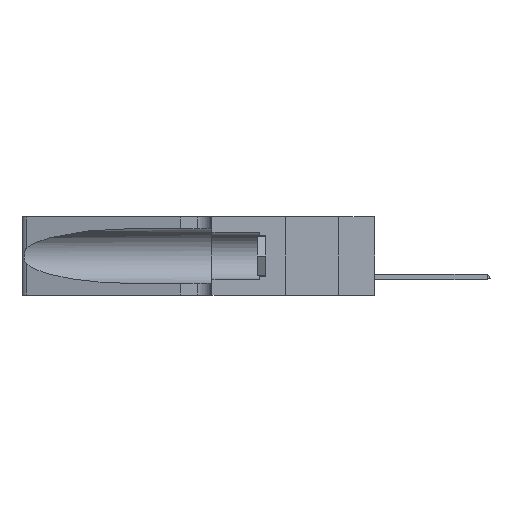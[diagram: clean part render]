
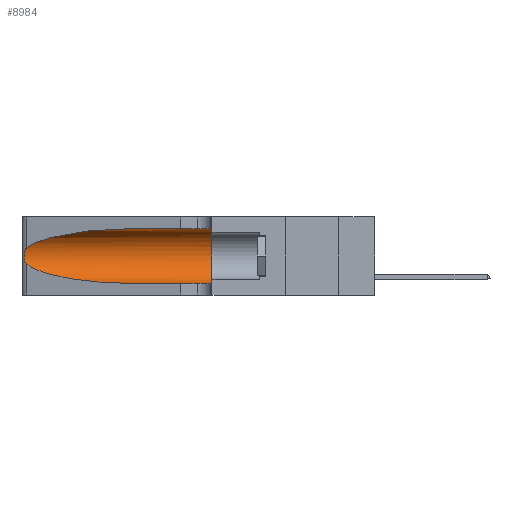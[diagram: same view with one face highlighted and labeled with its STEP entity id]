
A CAD part, left-side view. The second image highlights one B-rep face of the part: STEP entity #8984.
In plain terms, the highlighted cylindrical face has radius 3.308 mm (diameter 6.617 mm), a partial arc.
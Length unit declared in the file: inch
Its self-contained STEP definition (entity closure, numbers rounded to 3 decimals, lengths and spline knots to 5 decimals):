
#636 = EDGE_CURVE ( 'NONE', #5846, #15281, #7369, .T. ) ;
#882 = CARTESIAN_POINT ( 'NONE',  ( 0.25487, 1.22718, 0.14631 ) ) ;
#2503 = CARTESIAN_POINT ( 'NONE',  ( 0.26017, 1.23833, 0.17102 ) ) ;
#3140 = CARTESIAN_POINT ( 'NONE',  ( 0.1305, 0.72297, 0.31525 ) ) ;
#3546 = EDGE_CURVE ( 'NONE', #15281, #22573, #12371, .T. ) ;
#4072 = CYLINDRICAL_SURFACE ( 'NONE', #7129, 0.13025 ) ;
#5148 = CARTESIAN_POINT ( 'NONE',  ( 0.1305, 1.61858, 0.185 ) ) ;
#5846 = VERTEX_POINT ( 'NONE', #31992 ) ;
#6547 = DIRECTION ( 'NONE',  ( 0., 1., 0. ) ) ;
#7122 = EDGE_LOOP ( 'NONE', ( #8693, #24282, #16456, #20223, #13893, #24708 ) ) ;
#7129 = AXIS2_PLACEMENT_3D ( 'NONE', #5148, #10850, #8016 ) ;
#7369 =( BOUNDED_CURVE ( )  B_SPLINE_CURVE ( 3, ( #882, #25785, #34687, #11839 ),
 .UNSPECIFIED., .F., .F. ) 
 B_SPLINE_CURVE_WITH_KNOTS ( ( 4, 4 ),
 ( 3.44316, 4.71239 ),
 .UNSPECIFIED. ) 
 CURVE ( )  GEOMETRIC_REPRESENTATION_ITEM ( )  RATIONAL_B_SPLINE_CURVE ( ( 1., 0.87, 0.87, 1. ) ) 
 REPRESENTATION_ITEM ( '' )  );
#8016 = DIRECTION ( 'NONE',  ( 0., 0., -1. ) ) ;
#8693 = ORIENTED_EDGE ( 'NONE', *, *, #21580, .T. ) ;
#8801 = CARTESIAN_POINT ( 'NONE',  ( 0.18966, 0.96281, 0.31525 ) ) ;
#8984 = ADVANCED_FACE ( 'NONE', ( #14597 ), #4072, .F. ) ;
#9693 = CARTESIAN_POINT ( 'NONE',  ( 0.1305, 0.72297, 0.05475 ) ) ;
#9781 = CARTESIAN_POINT ( 'NONE',  ( 0.1305, 0.35, 0.05475 ) ) ;
#10850 = DIRECTION ( 'NONE',  ( 0., -1., 0. ) ) ;
#10878 = CARTESIAN_POINT ( 'NONE',  ( 0.26075, 1.23896, 0.19203 ) ) ;
#11839 = CARTESIAN_POINT ( 'NONE',  ( 0.1305, 0.72297, 0.05475 ) ) ;
#12362 = DIRECTION ( 'NONE',  ( 0., -1., 0. ) ) ;
#12371 = LINE ( 'NONE', #26182, #26880 ) ;
#12813 = CARTESIAN_POINT ( 'NONE',  ( 0.25787, 1.23484, 0.2124 ) ) ;
#13776 = CARTESIAN_POINT ( 'NONE',  ( 0.25789, 1.23486, 0.15765 ) ) ;
#13893 = ORIENTED_EDGE ( 'NONE', *, *, #22571, .F. ) ;
#14204 = EDGE_CURVE ( 'NONE', #33214, #27606, #22830, .T. ) ;
#14597 = FACE_OUTER_BOUND ( 'NONE', #7122, .T. ) ;
#15281 = VERTEX_POINT ( 'NONE', #9693 ) ;
#16448 = CIRCLE ( 'NONE', #31625, 0.13025 ) ;
#16456 = ORIENTED_EDGE ( 'NONE', *, *, #636, .T. ) ;
#17056 = DIRECTION ( 'NONE',  ( 0., -1., 0. ) ) ;
#17614 = CARTESIAN_POINT ( 'NONE',  ( 0.25487, 1.22718, 0.22369 ) ) ;
#18303 = CARTESIAN_POINT ( 'NONE',  ( 0.25639, 1.23184, 0.21858 ) ) ;
#19509 = CARTESIAN_POINT ( 'NONE',  ( 0.26018, 1.23835, 0.19895 ) ) ;
#20223 = ORIENTED_EDGE ( 'NONE', *, *, #3546, .T. ) ;
#20861 = CARTESIAN_POINT ( 'NONE',  ( 0.1305, 0.35, 0.185 ) ) ;
#21212 = CARTESIAN_POINT ( 'NONE',  ( 0.25555, 1.22994, 0.2215 ) ) ;
#21580 = EDGE_CURVE ( 'NONE', #33214, #31985, #34098, .T. ) ;
#22061 = CARTESIAN_POINT ( 'NONE',  ( 0.25487, 1.22718, 0.22369 ) ) ;
#22075 = CARTESIAN_POINT ( 'NONE',  ( 0.25856, 1.23593, 0.16098 ) ) ;
#22571 = EDGE_CURVE ( 'NONE', #27606, #22573, #16448, .T. ) ;
#22573 = VERTEX_POINT ( 'NONE', #9781 ) ;
#22830 = LINE ( 'NONE', #26149, #33499 ) ;
#23736 = DIRECTION ( 'NONE',  ( 0., 0., 1. ) ) ;
#23763 = EDGE_CURVE ( 'NONE', #31985, #5846, #31858, .T. ) ;
#24282 = ORIENTED_EDGE ( 'NONE', *, *, #23763, .T. ) ;
#24498 = CARTESIAN_POINT ( 'NONE',  ( 0.1305, 0.35, 0.31525 ) ) ;
#24708 = ORIENTED_EDGE ( 'NONE', *, *, #14204, .F. ) ;
#25785 = CARTESIAN_POINT ( 'NONE',  ( 0.2373, 1.15595, 0.08982 ) ) ;
#25991 = CARTESIAN_POINT ( 'NONE',  ( 0.25555, 1.22993, 0.14849 ) ) ;
#26149 = CARTESIAN_POINT ( 'NONE',  ( 0.1305, 1.61858, 0.31525 ) ) ;
#26182 = CARTESIAN_POINT ( 'NONE',  ( 0.1305, 1.61858, 0.05475 ) ) ;
#26254 = CARTESIAN_POINT ( 'NONE',  ( 0.25487, 1.22718, 0.14631 ) ) ;
#26880 = VECTOR ( 'NONE', #12362, 39.37008 ) ;
#27606 = VERTEX_POINT ( 'NONE', #24498 ) ;
#28343 = CARTESIAN_POINT ( 'NONE',  ( 0.25639, 1.23186, 0.15144 ) ) ;
#28419 = CARTESIAN_POINT ( 'NONE',  ( 0.2373, 1.15595, 0.28018 ) ) ;
#28789 = CARTESIAN_POINT ( 'NONE',  ( 0.1305, 0.72297, 0.31525 ) ) ;
#30496 = CARTESIAN_POINT ( 'NONE',  ( 0.26075, 1.23896, 0.178 ) ) ;
#31625 = AXIS2_PLACEMENT_3D ( 'NONE', #20861, #6547, #23736 ) ;
#31858 = B_SPLINE_CURVE_WITH_KNOTS ( 'NONE', 3,
 ( #32696, #21212, #18303, #12813, #32450, #19509, #10878, #30496, #2503, #22075, #13776, #28343, #25991, #26254 ),
 .UNSPECIFIED., .F., .F.,
 ( 4, 2, 2, 2, 2, 2, 4 ),
 ( 0., 0.00027, 0.00053, 0.00107, 0.0016, 0.00187, 0.00214 ),
 .UNSPECIFIED. ) ;
#31985 = VERTEX_POINT ( 'NONE', #22061 ) ;
#31992 = CARTESIAN_POINT ( 'NONE',  ( 0.25487, 1.22718, 0.14631 ) ) ;
#32450 = CARTESIAN_POINT ( 'NONE',  ( 0.25854, 1.2359, 0.20912 ) ) ;
#32696 = CARTESIAN_POINT ( 'NONE',  ( 0.25487, 1.22718, 0.22369 ) ) ;
#33214 = VERTEX_POINT ( 'NONE', #28789 ) ;
#33499 = VECTOR ( 'NONE', #17056, 39.37008 ) ;
#34098 =( BOUNDED_CURVE ( )  B_SPLINE_CURVE ( 3, ( #3140, #8801, #28419, #17614 ),
 .UNSPECIFIED., .F., .F. ) 
 B_SPLINE_CURVE_WITH_KNOTS ( ( 4, 4 ),
 ( 1.5708, 2.84003 ),
 .UNSPECIFIED. ) 
 CURVE ( )  GEOMETRIC_REPRESENTATION_ITEM ( )  RATIONAL_B_SPLINE_CURVE ( ( 1., 0.87, 0.87, 1. ) ) 
 REPRESENTATION_ITEM ( '' )  );
#34687 = CARTESIAN_POINT ( 'NONE',  ( 0.18966, 0.96281, 0.05475 ) ) ;
